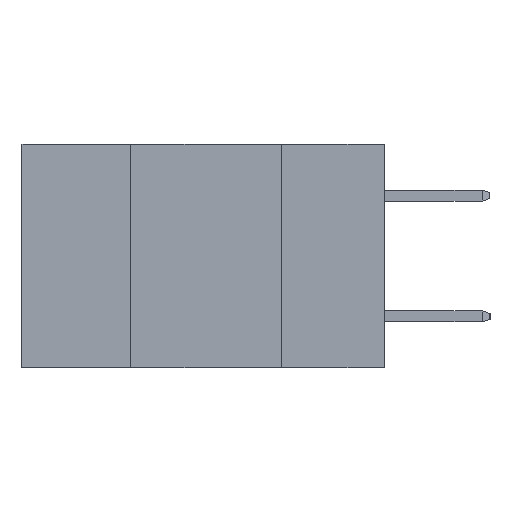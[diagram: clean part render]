
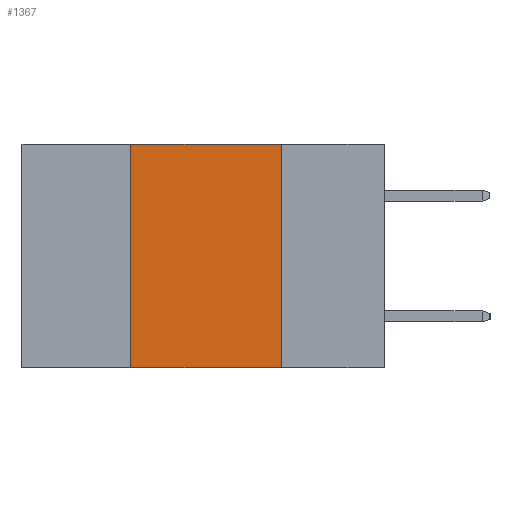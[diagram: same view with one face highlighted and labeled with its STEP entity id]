
A CAD part, left-side view. The second image highlights one B-rep face of the part: STEP entity #1367.
In plain terms, the highlighted planar face has unit normal (-1, 0, 0).
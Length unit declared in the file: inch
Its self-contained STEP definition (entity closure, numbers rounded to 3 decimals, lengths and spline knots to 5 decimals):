
#136 = DIRECTION ( 'NONE',  ( 0., 0., 1. ) ) ;
#458 = CARTESIAN_POINT ( 'NONE',  ( 0., 0.42, -0.37 ) ) ;
#543 = EDGE_LOOP ( 'NONE', ( #5854, #5820, #5758, #5696 ) ) ;
#805 = AXIS2_PLACEMENT_3D ( 'NONE', #8501, #1927, #1781 ) ;
#1094 = CARTESIAN_POINT ( 'NONE',  ( 0., 0.42, 0. ) ) ;
#1367 = ADVANCED_FACE ( 'NONE', ( #2117 ), #8301, .F. ) ;
#1400 = DIRECTION ( 'NONE',  ( 0., -1., 0. ) ) ;
#1502 = CARTESIAN_POINT ( 'NONE',  ( 0., 0.6, 0. ) ) ;
#1781 = DIRECTION ( 'NONE',  ( 0., 0., -1. ) ) ;
#1927 = DIRECTION ( 'NONE',  ( 1., 0., 0. ) ) ;
#1932 = LINE ( 'NONE', #1502, #7260 ) ;
#2117 = FACE_OUTER_BOUND ( 'NONE', #543, .T. ) ;
#2822 = CARTESIAN_POINT ( 'NONE',  ( 0., 0.6, -0.37 ) ) ;
#2989 = VECTOR ( 'NONE', #136, 39.37008 ) ;
#2995 = DIRECTION ( 'NONE',  ( 0., 0., -1. ) ) ;
#2999 = CARTESIAN_POINT ( 'NONE',  ( 0., 0.17, -0.37 ) ) ;
#3070 = VERTEX_POINT ( 'NONE', #5552 ) ;
#3318 = CARTESIAN_POINT ( 'NONE',  ( 0., 0.42, -0.37 ) ) ;
#3405 = LINE ( 'NONE', #2999, #6829 ) ;
#3516 = DIRECTION ( 'NONE',  ( 0., -1., 0. ) ) ;
#3636 = EDGE_CURVE ( 'NONE', #5535, #4631, #8141, .T. ) ;
#3672 = VECTOR ( 'NONE', #3516, 39.37008 ) ;
#4090 = EDGE_CURVE ( 'NONE', #4631, #5375, #1932, .T. ) ;
#4514 = EDGE_CURVE ( 'NONE', #5375, #3070, #3405, .T. ) ;
#4631 = VERTEX_POINT ( 'NONE', #1094 ) ;
#5375 = VERTEX_POINT ( 'NONE', #6704 ) ;
#5535 = VERTEX_POINT ( 'NONE', #3318 ) ;
#5552 = CARTESIAN_POINT ( 'NONE',  ( 0., 0.17, -0.37 ) ) ;
#5696 = ORIENTED_EDGE ( 'NONE', *, *, #8104, .T. ) ;
#5758 = ORIENTED_EDGE ( 'NONE', *, *, #3636, .F. ) ;
#5820 = ORIENTED_EDGE ( 'NONE', *, *, #4090, .F. ) ;
#5854 = ORIENTED_EDGE ( 'NONE', *, *, #4514, .F. ) ;
#6704 = CARTESIAN_POINT ( 'NONE',  ( 0., 0.17, 0. ) ) ;
#6829 = VECTOR ( 'NONE', #2995, 39.37008 ) ;
#7260 = VECTOR ( 'NONE', #1400, 39.37008 ) ;
#8104 = EDGE_CURVE ( 'NONE', #5535, #3070, #8727, .T. ) ;
#8141 = LINE ( 'NONE', #458, #2989 ) ;
#8301 = PLANE ( 'NONE',  #805 ) ;
#8501 = CARTESIAN_POINT ( 'NONE',  ( 0., 0.6, 0. ) ) ;
#8727 = LINE ( 'NONE', #2822, #3672 ) ;
